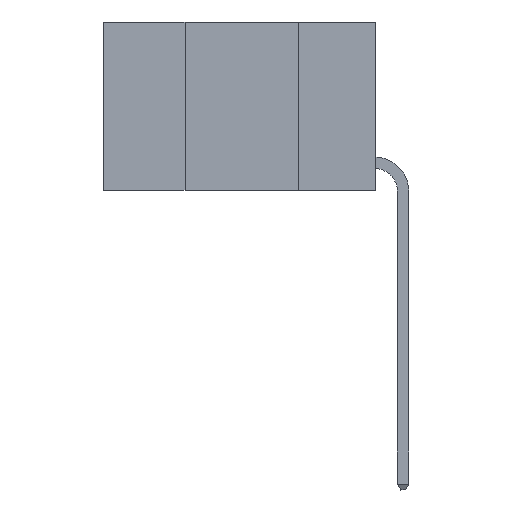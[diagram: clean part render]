
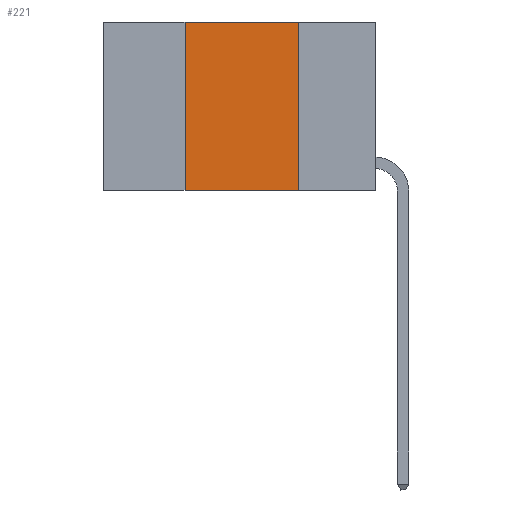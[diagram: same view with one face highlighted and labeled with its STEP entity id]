
A CAD part, left-side view. The second image highlights one B-rep face of the part: STEP entity #221.
In plain terms, the highlighted planar face has unit normal (-1, 0, 0).
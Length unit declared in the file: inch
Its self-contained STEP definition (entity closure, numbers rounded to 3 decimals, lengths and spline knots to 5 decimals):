
#175 = ORIENTED_EDGE ( 'NONE', *, *, #7242, .F. ) ;
#221 = ADVANCED_FACE ( 'NONE', ( #11262 ), #11507, .F. ) ;
#333 = EDGE_LOOP ( 'NONE', ( #1427, #175, #2346, #10704 ) ) ;
#421 = DIRECTION ( 'NONE',  ( 0., 0., -1. ) ) ;
#1125 = LINE ( 'NONE', #7216, #6015 ) ;
#1354 = DIRECTION ( 'NONE',  ( 0., -1., 0. ) ) ;
#1427 = ORIENTED_EDGE ( 'NONE', *, *, #9083, .F. ) ;
#1563 = VERTEX_POINT ( 'NONE', #7872 ) ;
#2346 = ORIENTED_EDGE ( 'NONE', *, *, #3181, .F. ) ;
#2938 = VERTEX_POINT ( 'NONE', #12111 ) ;
#3181 = EDGE_CURVE ( 'NONE', #10096, #2938, #12075, .T. ) ;
#3912 = DIRECTION ( 'NONE',  ( 0., 0., 1. ) ) ;
#4409 = DIRECTION ( 'NONE',  ( 0., -1., 0. ) ) ;
#4534 = CARTESIAN_POINT ( 'NONE',  ( 0., 0.6, 0. ) ) ;
#4611 = CARTESIAN_POINT ( 'NONE',  ( 0., 0.42, 0. ) ) ;
#5190 = EDGE_CURVE ( 'NONE', #10096, #1563, #1125, .T. ) ;
#6015 = VECTOR ( 'NONE', #1354, 39.37008 ) ;
#6286 = CARTESIAN_POINT ( 'NONE',  ( 0., 0.17, 0. ) ) ;
#6717 = VERTEX_POINT ( 'NONE', #10306 ) ;
#7216 = CARTESIAN_POINT ( 'NONE',  ( 0., 0.6, -0.37 ) ) ;
#7242 = EDGE_CURVE ( 'NONE', #2938, #6717, #12123, .T. ) ;
#7290 = VECTOR ( 'NONE', #3912, 39.37008 ) ;
#7305 = VECTOR ( 'NONE', #421, 39.37008 ) ;
#7375 = DIRECTION ( 'NONE',  ( 0., 0., -1. ) ) ;
#7593 = LINE ( 'NONE', #6286, #7305 ) ;
#7872 = CARTESIAN_POINT ( 'NONE',  ( 0., 0.17, -0.37 ) ) ;
#8828 = CARTESIAN_POINT ( 'NONE',  ( 0., 0.42, -0.37 ) ) ;
#9083 = EDGE_CURVE ( 'NONE', #6717, #1563, #7593, .T. ) ;
#9870 = VECTOR ( 'NONE', #4409, 39.37008 ) ;
#10096 = VERTEX_POINT ( 'NONE', #8828 ) ;
#10226 = DIRECTION ( 'NONE',  ( 1., 0., 0. ) ) ;
#10306 = CARTESIAN_POINT ( 'NONE',  ( 0., 0.17, 0. ) ) ;
#10704 = ORIENTED_EDGE ( 'NONE', *, *, #5190, .T. ) ;
#11029 = CARTESIAN_POINT ( 'NONE',  ( 0., 0.6, 0. ) ) ;
#11066 = AXIS2_PLACEMENT_3D ( 'NONE', #4534, #10226, #7375 ) ;
#11262 = FACE_OUTER_BOUND ( 'NONE', #333, .T. ) ;
#11507 = PLANE ( 'NONE',  #11066 ) ;
#12075 = LINE ( 'NONE', #4611, #7290 ) ;
#12111 = CARTESIAN_POINT ( 'NONE',  ( 0., 0.42, 0. ) ) ;
#12123 = LINE ( 'NONE', #11029, #9870 ) ;
